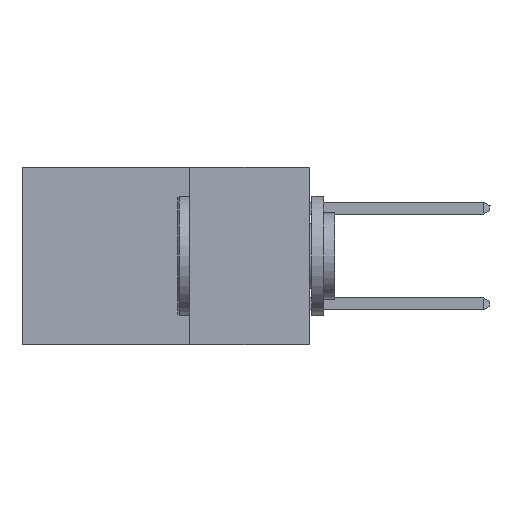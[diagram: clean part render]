
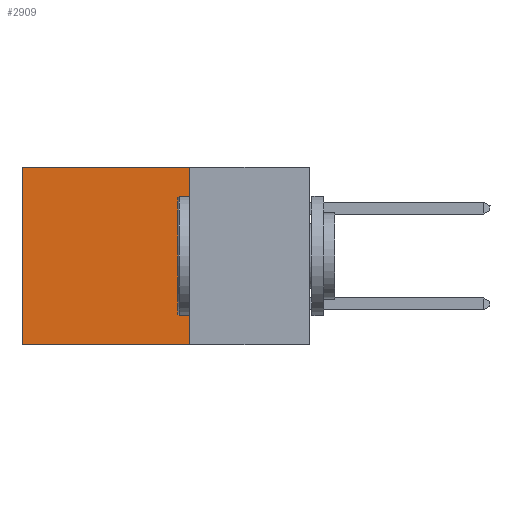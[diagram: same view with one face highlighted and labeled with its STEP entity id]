
A CAD part, left-side view. The second image highlights one B-rep face of the part: STEP entity #2909.
In plain terms, the highlighted planar face has unit normal (-1, 0, 0).
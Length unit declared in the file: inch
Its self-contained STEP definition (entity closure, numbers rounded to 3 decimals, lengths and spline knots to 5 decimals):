
#414 = CARTESIAN_POINT ( 'NONE',  ( 0.2875, 0.25, -0.37 ) ) ;
#708 = ORIENTED_EDGE ( 'NONE', *, *, #5750, .F. ) ;
#879 = EDGE_CURVE ( 'NONE', #7296, #20043, #22580, .T. ) ;
#1201 = FACE_OUTER_BOUND ( 'NONE', #10591, .T. ) ;
#1273 = DIRECTION ( 'NONE',  ( 0., 1., 0. ) ) ;
#1585 = ORIENTED_EDGE ( 'NONE', *, *, #6332, .T. ) ;
#1955 = CARTESIAN_POINT ( 'NONE',  ( 0.2875, 0.25, 0. ) ) ;
#2248 = DIRECTION ( 'NONE',  ( 1., 0., 0. ) ) ;
#2290 = PLANE ( 'NONE',  #15598 ) ;
#2437 = DIRECTION ( 'NONE',  ( 0., 0., -1. ) ) ;
#2909 = ADVANCED_FACE ( 'NONE', ( #1201 ), #2290, .F. ) ;
#3031 = CARTESIAN_POINT ( 'NONE',  ( 0.2875, 0.25, -0.37 ) ) ;
#3072 = CARTESIAN_POINT ( 'NONE',  ( 0.2875, 0.25, 0. ) ) ;
#3868 = VECTOR ( 'NONE', #13323, 39.37008 ) ;
#4029 = ORIENTED_EDGE ( 'NONE', *, *, #879, .F. ) ;
#4237 = VECTOR ( 'NONE', #5589, 39.37008 ) ;
#4956 = VERTEX_POINT ( 'NONE', #9951 ) ;
#5589 = DIRECTION ( 'NONE',  ( 0., 0., -1. ) ) ;
#5604 = LINE ( 'NONE', #11595, #3868 ) ;
#5750 = EDGE_CURVE ( 'NONE', #20043, #20054, #19927, .T. ) ;
#6332 = EDGE_CURVE ( 'NONE', #7296, #4956, #5604, .T. ) ;
#7296 = VERTEX_POINT ( 'NONE', #3072 ) ;
#9142 = CARTESIAN_POINT ( 'NONE',  ( 0.2875, 0.25, 0. ) ) ;
#9951 = CARTESIAN_POINT ( 'NONE',  ( 0.2875, 0.6, 0. ) ) ;
#10591 = EDGE_LOOP ( 'NONE', ( #14864, #708, #4029, #1585 ) ) ;
#10806 = VECTOR ( 'NONE', #1273, 39.37008 ) ;
#11101 = CARTESIAN_POINT ( 'NONE',  ( 0.2875, 0.6, -0.37 ) ) ;
#11595 = CARTESIAN_POINT ( 'NONE',  ( 0.2875, 0.25, 0. ) ) ;
#13009 = LINE ( 'NONE', #18609, #17061 ) ;
#13323 = DIRECTION ( 'NONE',  ( 0., 1., 0. ) ) ;
#14864 = ORIENTED_EDGE ( 'NONE', *, *, #16384, .T. ) ;
#15598 = AXIS2_PLACEMENT_3D ( 'NONE', #1955, #2248, #2437 ) ;
#16384 = EDGE_CURVE ( 'NONE', #4956, #20054, #13009, .T. ) ;
#17061 = VECTOR ( 'NONE', #20310, 39.37008 ) ;
#18609 = CARTESIAN_POINT ( 'NONE',  ( 0.2875, 0.6, 0. ) ) ;
#19927 = LINE ( 'NONE', #3031, #10806 ) ;
#20043 = VERTEX_POINT ( 'NONE', #414 ) ;
#20054 = VERTEX_POINT ( 'NONE', #11101 ) ;
#20310 = DIRECTION ( 'NONE',  ( 0., 0., -1. ) ) ;
#22580 = LINE ( 'NONE', #9142, #4237 ) ;
